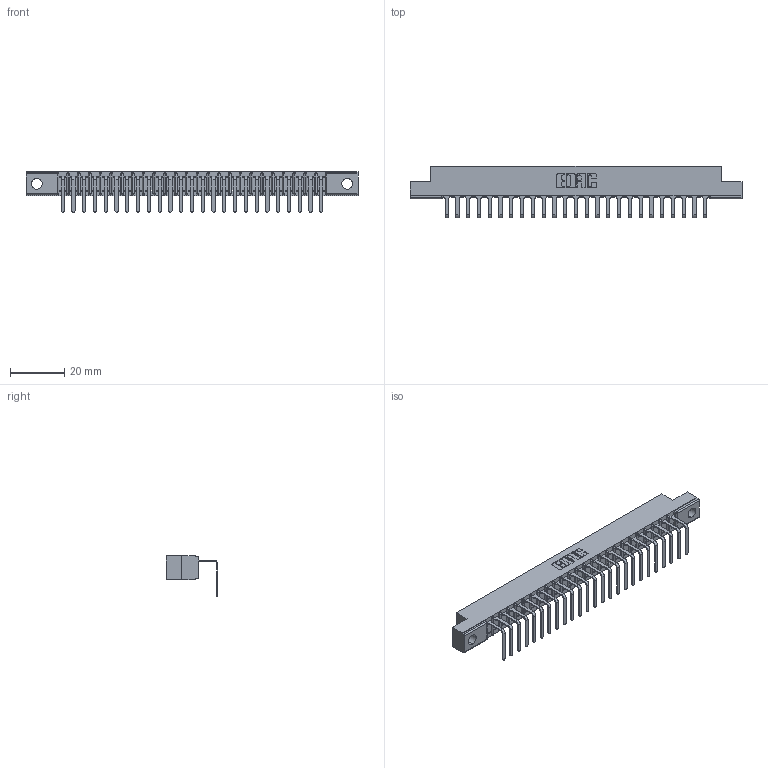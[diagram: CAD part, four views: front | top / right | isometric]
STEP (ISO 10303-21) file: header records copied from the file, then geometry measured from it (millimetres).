
FILE_DESCRIPTION (( 'STEP AP203' ), '1' );
FILE_NAME ('307-025-558-104.STEP', '2019-09-04T13:48:26', ( '' ), ( '' ), 'SwSTEP 2.0', 'SolidWorks 2016', '' );
FILE_SCHEMA (( 'CONFIG_CONTROL_DESIGN' ));
Length unit declared in the file: inch
Products named in the file (3): 307-290-001_558 - 2 (Single); 307-025-558-104; 307 Part_.156 Dia Mounting Holes
Assembly tree (26 placements, depth 2):
  307-025-558-104
    307 Part_.156 Dia Mounting Holes
    307-290-001_558 - 2 (Single)  x25
Bounding box: 122.07 x 18.96 x 14.81 mm (x, y, z)
Volume: 7707.1 mm3; surface area: 12618.5 mm2
Topology: 26 solids, 26 shells, 1658 faces, 4709 edges, 3034 vertices
Faces by surface type: plane 1059, cylinder 547, sphere 52
Entity records: 24050 total; most frequent: CARTESIAN_POINT 4050, ORIENTED_EDGE 4034, DIRECTION 3941, EDGE_CURVE 2017, VECTOR 1547, LINE 1547, VERTEX_POINT 1306, AXIS2_PLACEMENT_3D 1197
